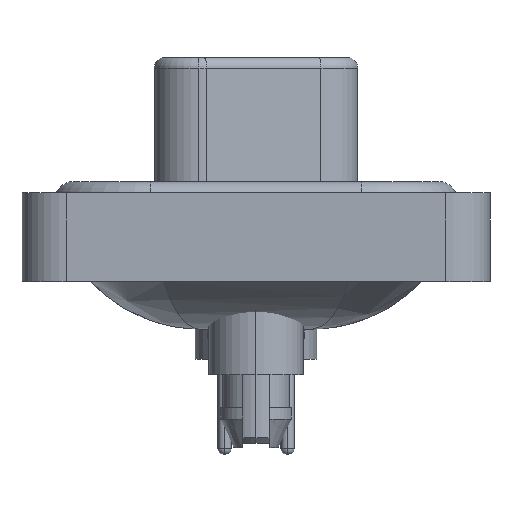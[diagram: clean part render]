
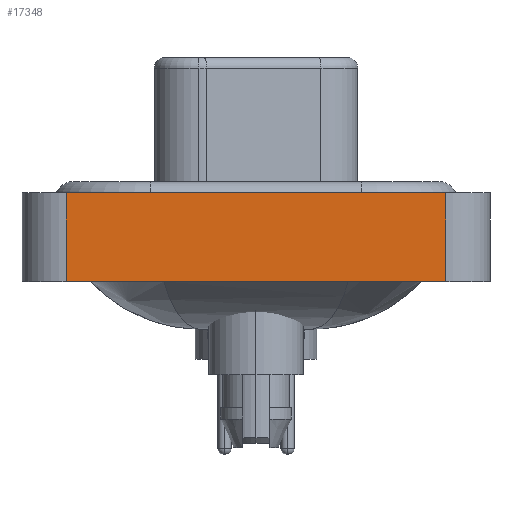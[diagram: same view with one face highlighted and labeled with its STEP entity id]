
A CAD part, left-side view. The second image highlights one B-rep face of the part: STEP entity #17348.
In plain terms, the highlighted planar face has unit normal (-1, 0, 0).
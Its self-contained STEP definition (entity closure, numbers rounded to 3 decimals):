
#159 = LINE ( 'NONE', #15260, #15399 ) ;
#741 = FACE_OUTER_BOUND ( 'NONE', #20913, .T. ) ;
#933 = VERTEX_POINT ( 'NONE', #10876 ) ;
#1726 = LINE ( 'NONE', #5149, #9081 ) ;
#2310 = VERTEX_POINT ( 'NONE', #3178 ) ;
#2731 = CARTESIAN_POINT ( 'NONE',  ( -7.3, 8.55, -3.6 ) ) ;
#2892 = EDGE_CURVE ( 'NONE', #933, #2310, #17800, .T. ) ;
#3144 = DIRECTION ( 'NONE',  ( 0., 0., 1. ) ) ;
#3178 = CARTESIAN_POINT ( 'NONE',  ( -7.3, 8.55, 0.4 ) ) ;
#3517 = AXIS2_PLACEMENT_3D ( 'NONE', #21469, #18000, #3144 ) ;
#3590 = DIRECTION ( 'NONE',  ( 0., -1., 0. ) ) ;
#5149 = CARTESIAN_POINT ( 'NONE',  ( -7.3, -8.55, -3.6 ) ) ;
#6181 = EDGE_CURVE ( 'NONE', #933, #20125, #1726, .T. ) ;
#7131 = VECTOR ( 'NONE', #12375, 1000. ) ;
#7412 = ORIENTED_EDGE ( 'NONE', *, *, #6181, .T. ) ;
#7426 = LINE ( 'NONE', #15299, #7131 ) ;
#7431 = PLANE ( 'NONE',  #3517 ) ;
#9081 = VECTOR ( 'NONE', #3590, 1000. ) ;
#10026 = EDGE_CURVE ( 'NONE', #2310, #17577, #159, .T. ) ;
#10289 = CARTESIAN_POINT ( 'NONE',  ( -7.3, -8.55, -3.6 ) ) ;
#10876 = CARTESIAN_POINT ( 'NONE',  ( -7.3, 8.55, -3.6 ) ) ;
#12375 = DIRECTION ( 'NONE',  ( 0., 0., 1. ) ) ;
#12860 = ORIENTED_EDGE ( 'NONE', *, *, #21482, .T. ) ;
#13148 = VECTOR ( 'NONE', #14559, 1000. ) ;
#13531 = DIRECTION ( 'NONE',  ( 0., -1., 0. ) ) ;
#13646 = CARTESIAN_POINT ( 'NONE',  ( -7.3, -8.55, 0.4 ) ) ;
#14559 = DIRECTION ( 'NONE',  ( 0., 0., 1. ) ) ;
#15260 = CARTESIAN_POINT ( 'NONE',  ( -7.3, -8.55, 0.4 ) ) ;
#15299 = CARTESIAN_POINT ( 'NONE',  ( -7.3, -8.55, -3.6 ) ) ;
#15399 = VECTOR ( 'NONE', #13531, 1000. ) ;
#16864 = ORIENTED_EDGE ( 'NONE', *, *, #10026, .F. ) ;
#17348 = ADVANCED_FACE ( 'NONE', ( #741 ), #7431, .T. ) ;
#17577 = VERTEX_POINT ( 'NONE', #13646 ) ;
#17800 = LINE ( 'NONE', #2731, #13148 ) ;
#18000 = DIRECTION ( 'NONE',  ( -1., 0., 0. ) ) ;
#18971 = ORIENTED_EDGE ( 'NONE', *, *, #2892, .F. ) ;
#20125 = VERTEX_POINT ( 'NONE', #10289 ) ;
#20913 = EDGE_LOOP ( 'NONE', ( #12860, #16864, #18971, #7412 ) ) ;
#21469 = CARTESIAN_POINT ( 'NONE',  ( -7.3, -8.55, -3.6 ) ) ;
#21482 = EDGE_CURVE ( 'NONE', #20125, #17577, #7426, .T. ) ;
